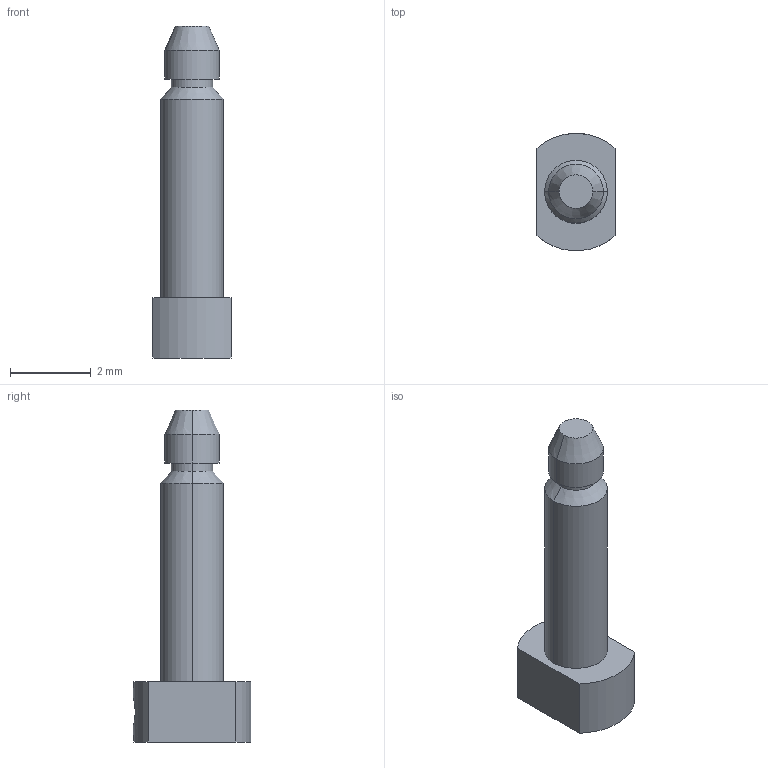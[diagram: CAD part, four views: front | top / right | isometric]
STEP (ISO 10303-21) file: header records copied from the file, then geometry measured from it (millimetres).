
FILE_DESCRIPTION (( 'STEP AP214' ), '1' );
FILE_NAME ('565-200-100.STEP', '2020-09-17T17:35:02', ( '' ), ( '' ), 'SwSTEP 2.0', 'SolidWorks 2020', '' );
FILE_SCHEMA (( 'AUTOMOTIVE_DESIGN' ));
Length unit declared in the file: millimetre
Products named in the file (1): 565-200-100
Bounding box: 1.93 x 2.9 x 8.2 mm (x, y, z)
Volume: 18.6 mm3; surface area: 55.3 mm2
Topology: 1 solids, 1 shells, 25 faces, 51 edges, 32 vertices
Faces by surface type: cylinder 10, plane 8, cone 7
Entity records: 711 total; most frequent: CARTESIAN_POINT 127, DIRECTION 127, ORIENTED_EDGE 102, AXIS2_PLACEMENT_3D 52, EDGE_CURVE 51, VERTEX_POINT 32, EDGE_LOOP 29, CIRCLE 26
